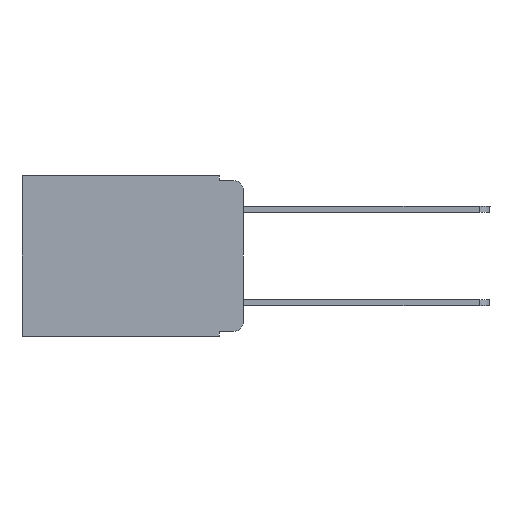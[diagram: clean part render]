
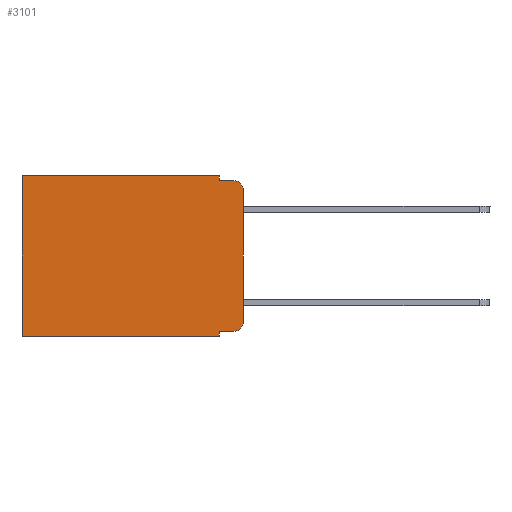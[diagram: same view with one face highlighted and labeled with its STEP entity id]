
A CAD part, left-side view. The second image highlights one B-rep face of the part: STEP entity #3101.
In plain terms, the highlighted planar face has unit normal (-1, 0, 0).
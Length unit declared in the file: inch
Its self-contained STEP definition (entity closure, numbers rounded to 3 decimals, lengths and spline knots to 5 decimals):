
#429 = CIRCLE ( 'NONE', #8229, 0.02 ) ;
#516 = CARTESIAN_POINT ( 'NONE',  ( 0.298, 0.051, -0.333 ) ) ;
#1324 = CARTESIAN_POINT ( 'NONE',  ( 0.298, 0.051, -0.01 ) ) ;
#1562 = LINE ( 'NONE', #7747, #3961 ) ;
#1579 = CARTESIAN_POINT ( 'NONE',  ( 0.298, 0.473, -0.343 ) ) ;
#1869 = DIRECTION ( 'NONE',  ( 0., 0., -1. ) ) ;
#2068 = VECTOR ( 'NONE', #11037, 39.37008 ) ;
#2204 = CARTESIAN_POINT ( 'NONE',  ( 0.298, 0.473, 0. ) ) ;
#3101 = ADVANCED_FACE ( 'NONE', ( #12648 ), #11224, .F. ) ;
#3682 = LINE ( 'NONE', #14813, #14972 ) ;
#3744 = VERTEX_POINT ( 'NONE', #5009 ) ;
#3879 = VERTEX_POINT ( 'NONE', #5416 ) ;
#3961 = VECTOR ( 'NONE', #14022, 39.37008 ) ;
#4171 = EDGE_CURVE ( 'NONE', #15446, #6318, #11330, .T. ) ;
#4413 = ORIENTED_EDGE ( 'NONE', *, *, #15772, .T. ) ;
#4604 = CIRCLE ( 'NONE', #14732, 0.02 ) ;
#4826 = ORIENTED_EDGE ( 'NONE', *, *, #19990, .F. ) ;
#4908 = CARTESIAN_POINT ( 'NONE',  ( 0.298, 0.051, 0. ) ) ;
#5009 = CARTESIAN_POINT ( 'NONE',  ( 0.298, 0., -0.313 ) ) ;
#5416 = CARTESIAN_POINT ( 'NONE',  ( 0.298, 0.051, -0.343 ) ) ;
#5470 = ORIENTED_EDGE ( 'NONE', *, *, #17770, .F. ) ;
#6318 = VERTEX_POINT ( 'NONE', #1579 ) ;
#6355 = CARTESIAN_POINT ( 'NONE',  ( 0.298, 0.051, 0. ) ) ;
#6423 = LINE ( 'NONE', #15871, #16764 ) ;
#6573 = DIRECTION ( 'NONE',  ( 0., 0., -1. ) ) ;
#6614 = ORIENTED_EDGE ( 'NONE', *, *, #14101, .T. ) ;
#6800 = EDGE_LOOP ( 'NONE', ( #10518, #4413, #4826, #5470, #12459, #16727, #13585, #10536, #6614, #6883 ) ) ;
#6883 = ORIENTED_EDGE ( 'NONE', *, *, #19838, .T. ) ;
#6973 = DIRECTION ( 'NONE',  ( 0., -1., 0. ) ) ;
#7041 = LINE ( 'NONE', #516, #10752 ) ;
#7714 = DIRECTION ( 'NONE',  ( 0., 0., -1. ) ) ;
#7747 = CARTESIAN_POINT ( 'NONE',  ( 0.298, 0., 0. ) ) ;
#8012 = CARTESIAN_POINT ( 'NONE',  ( 0.298, 0.473, 0. ) ) ;
#8229 = AXIS2_PLACEMENT_3D ( 'NONE', #13788, #17634, #10913 ) ;
#9304 = DIRECTION ( 'NONE',  ( 0., 0., -1. ) ) ;
#9648 = CARTESIAN_POINT ( 'NONE',  ( 0.298, 0., -0.03 ) ) ;
#10065 = DIRECTION ( 'NONE',  ( 1., 0., 0. ) ) ;
#10136 = CARTESIAN_POINT ( 'NONE',  ( 0.298, 0.02, -0.01 ) ) ;
#10281 = CARTESIAN_POINT ( 'NONE',  ( 0.298, 0., 0. ) ) ;
#10518 = ORIENTED_EDGE ( 'NONE', *, *, #17067, .F. ) ;
#10536 = ORIENTED_EDGE ( 'NONE', *, *, #19417, .F. ) ;
#10749 = LINE ( 'NONE', #4908, #2068 ) ;
#10752 = VECTOR ( 'NONE', #11581, 39.37008 ) ;
#10853 = CARTESIAN_POINT ( 'NONE',  ( 0.298, 0.02, -0.03 ) ) ;
#10913 = DIRECTION ( 'NONE',  ( 0., 0., -1. ) ) ;
#11037 = DIRECTION ( 'NONE',  ( 0., 0., -1. ) ) ;
#11224 = PLANE ( 'NONE',  #14445 ) ;
#11330 = LINE ( 'NONE', #8012, #17498 ) ;
#11439 = VERTEX_POINT ( 'NONE', #6355 ) ;
#11581 = DIRECTION ( 'NONE',  ( 0., -1., 0. ) ) ;
#12236 = CARTESIAN_POINT ( 'NONE',  ( 0.298, 0.051, -0.333 ) ) ;
#12459 = ORIENTED_EDGE ( 'NONE', *, *, #15783, .T. ) ;
#12648 = FACE_OUTER_BOUND ( 'NONE', #6800, .T. ) ;
#13215 = EDGE_CURVE ( 'NONE', #3879, #6318, #3682, .T. ) ;
#13585 = ORIENTED_EDGE ( 'NONE', *, *, #13215, .F. ) ;
#13603 = VERTEX_POINT ( 'NONE', #12236 ) ;
#13734 = VERTEX_POINT ( 'NONE', #9648 ) ;
#13788 = CARTESIAN_POINT ( 'NONE',  ( 0.298, 0.02, -0.313 ) ) ;
#14022 = DIRECTION ( 'NONE',  ( 0., 1., 0. ) ) ;
#14101 = EDGE_CURVE ( 'NONE', #13603, #14678, #7041, .T. ) ;
#14394 = DIRECTION ( 'NONE',  ( 0., 1., 0. ) ) ;
#14412 = VERTEX_POINT ( 'NONE', #15849 ) ;
#14445 = AXIS2_PLACEMENT_3D ( 'NONE', #17460, #10065, #6573 ) ;
#14678 = VERTEX_POINT ( 'NONE', #19718 ) ;
#14732 = AXIS2_PLACEMENT_3D ( 'NONE', #10853, #19965, #9304 ) ;
#14813 = CARTESIAN_POINT ( 'NONE',  ( 0.298, 0., -0.343 ) ) ;
#14972 = VECTOR ( 'NONE', #14394, 39.37008 ) ;
#15321 = LINE ( 'NONE', #1324, #17756 ) ;
#15405 = VECTOR ( 'NONE', #16445, 39.37008 ) ;
#15446 = VERTEX_POINT ( 'NONE', #2204 ) ;
#15772 = EDGE_CURVE ( 'NONE', #13734, #19213, #4604, .T. ) ;
#15783 = EDGE_CURVE ( 'NONE', #11439, #15446, #1562, .T. ) ;
#15849 = CARTESIAN_POINT ( 'NONE',  ( 0.298, 0.051, -0.01 ) ) ;
#15871 = CARTESIAN_POINT ( 'NONE',  ( 0.298, 0.051, 0. ) ) ;
#16445 = DIRECTION ( 'NONE',  ( 0., 0., -1. ) ) ;
#16727 = ORIENTED_EDGE ( 'NONE', *, *, #4171, .T. ) ;
#16764 = VECTOR ( 'NONE', #1869, 39.37008 ) ;
#17067 = EDGE_CURVE ( 'NONE', #13734, #3744, #19189, .T. ) ;
#17460 = CARTESIAN_POINT ( 'NONE',  ( 0.298, 0., 0. ) ) ;
#17498 = VECTOR ( 'NONE', #7714, 39.37008 ) ;
#17634 = DIRECTION ( 'NONE',  ( -1., 0., 0. ) ) ;
#17756 = VECTOR ( 'NONE', #6973, 39.37008 ) ;
#17770 = EDGE_CURVE ( 'NONE', #11439, #14412, #6423, .T. ) ;
#19189 = LINE ( 'NONE', #10281, #15405 ) ;
#19213 = VERTEX_POINT ( 'NONE', #10136 ) ;
#19417 = EDGE_CURVE ( 'NONE', #13603, #3879, #10749, .T. ) ;
#19718 = CARTESIAN_POINT ( 'NONE',  ( 0.298, 0.02, -0.333 ) ) ;
#19838 = EDGE_CURVE ( 'NONE', #14678, #3744, #429, .T. ) ;
#19965 = DIRECTION ( 'NONE',  ( -1., 0., 0. ) ) ;
#19990 = EDGE_CURVE ( 'NONE', #14412, #19213, #15321, .T. ) ;
